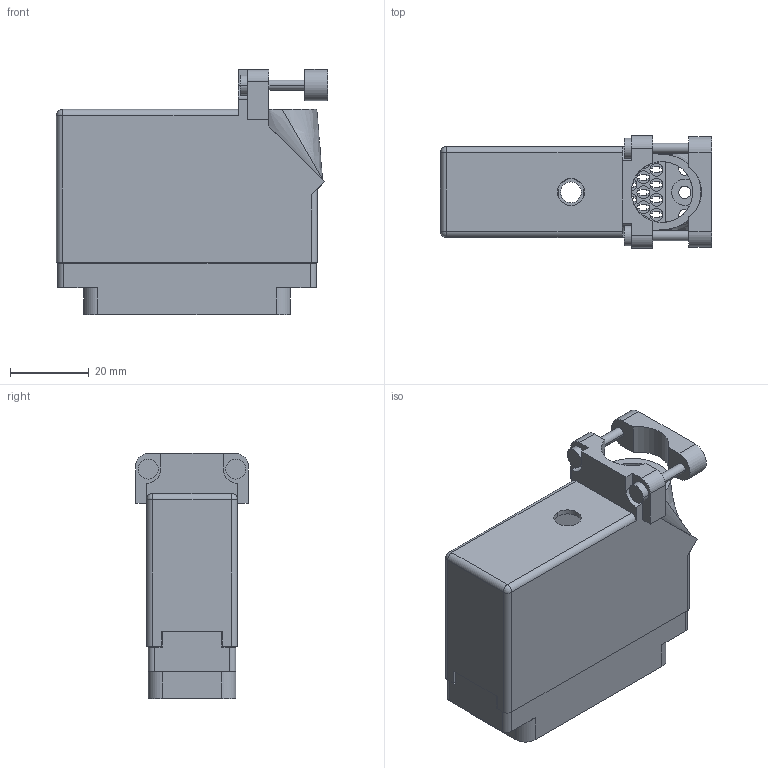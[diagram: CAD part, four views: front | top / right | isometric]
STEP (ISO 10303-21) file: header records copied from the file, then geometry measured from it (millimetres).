
FILE_DESCRIPTION (( 'STEP AP203' ), '1' );
FILE_NAME ('516-056-000-530.STEP', '2020-03-10T05:10:53', ( '' ), ( '' ), 'SwSTEP 2.0', 'SolidWorks 2016', '' );
FILE_SCHEMA (( 'CONFIG_CONTROL_DESIGN' ));
Length unit declared in the file: inch
Products named in the file (3): 516 Plug Insulator_056; 516-230-001_Plastic - 056 Top Entry - Large Clamp; 516-056-000-530
Assembly tree (2 placements, depth 2):
  516-056-000-530
    516 Plug Insulator_056
    516-230-001_Plastic - 056 Top Entry - Large Clamp
Bounding box: 68.91 x 28.57 x 62.28 mm (x, y, z)
Volume: 24281.7 mm3; surface area: 32614.9 mm2
Topology: 2 solids, 2 shells, 1299 faces, 3814 edges, 2538 vertices
Faces by surface type: plane 942, cylinder 350, bspline 3, cone 2, sphere 2
Entity records: 43776 total; most frequent: CARTESIAN_POINT 7747, ORIENTED_EDGE 7624, DIRECTION 7333, EDGE_CURVE 3812, VECTOR 2885, LINE 2885, VERTEX_POINT 2538, AXIS2_PLACEMENT_3D 2224
